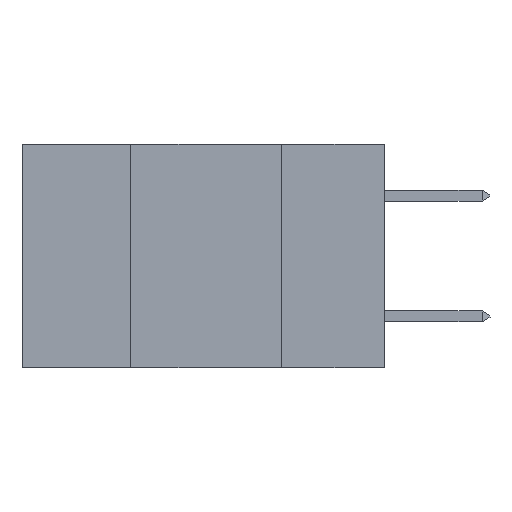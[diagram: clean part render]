
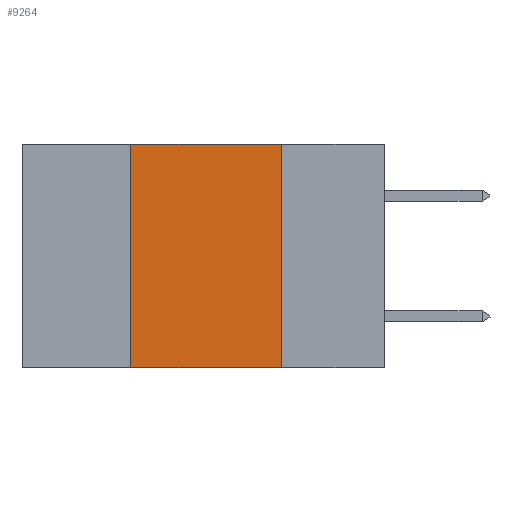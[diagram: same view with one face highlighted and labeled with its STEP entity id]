
A CAD part, left-side view. The second image highlights one B-rep face of the part: STEP entity #9264.
In plain terms, the highlighted planar face has unit normal (-1, 0, 0).
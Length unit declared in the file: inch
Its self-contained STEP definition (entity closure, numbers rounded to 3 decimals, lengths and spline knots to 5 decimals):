
#199 = ORIENTED_EDGE ( 'NONE', *, *, #4624, .F. ) ;
#1843 = CARTESIAN_POINT ( 'NONE',  ( 0., 0.6, 0. ) ) ;
#1872 = CARTESIAN_POINT ( 'NONE',  ( 0., 0.6, 0. ) ) ;
#2450 = VERTEX_POINT ( 'NONE', #16809 ) ;
#3179 = VECTOR ( 'NONE', #14970, 39.37008 ) ;
#3286 = ORIENTED_EDGE ( 'NONE', *, *, #17825, .F. ) ;
#4027 = LINE ( 'NONE', #6583, #3179 ) ;
#4624 = EDGE_CURVE ( 'NONE', #12736, #6586, #13359, .T. ) ;
#4851 = EDGE_CURVE ( 'NONE', #12736, #7540, #17727, .T. ) ;
#5351 = CARTESIAN_POINT ( 'NONE',  ( 0., 0.17, -0.37 ) ) ;
#5704 = LINE ( 'NONE', #1872, #9385 ) ;
#6222 = PLANE ( 'NONE',  #11294 ) ;
#6583 = CARTESIAN_POINT ( 'NONE',  ( 0., 0.17, 0. ) ) ;
#6586 = VERTEX_POINT ( 'NONE', #15947 ) ;
#6644 = CARTESIAN_POINT ( 'NONE',  ( 0., 0.6, -0.37 ) ) ;
#7540 = VERTEX_POINT ( 'NONE', #5351 ) ;
#7575 = DIRECTION ( 'NONE',  ( 0., 0., -1. ) ) ;
#7886 = DIRECTION ( 'NONE',  ( 0., 0., 1. ) ) ;
#8541 = CARTESIAN_POINT ( 'NONE',  ( 0., 0.42, 0. ) ) ;
#8892 = DIRECTION ( 'NONE',  ( 0., -1., 0. ) ) ;
#9264 = ADVANCED_FACE ( 'NONE', ( #11070 ), #6222, .F. ) ;
#9385 = VECTOR ( 'NONE', #8892, 39.37008 ) ;
#9632 = VECTOR ( 'NONE', #7886, 39.37008 ) ;
#9831 = VECTOR ( 'NONE', #15040, 39.37008 ) ;
#11070 = FACE_OUTER_BOUND ( 'NONE', #12857, .T. ) ;
#11294 = AXIS2_PLACEMENT_3D ( 'NONE', #1843, #15993, #7575 ) ;
#11961 = ORIENTED_EDGE ( 'NONE', *, *, #4851, .T. ) ;
#12736 = VERTEX_POINT ( 'NONE', #14483 ) ;
#12766 = EDGE_CURVE ( 'NONE', #6586, #2450, #5704, .T. ) ;
#12857 = EDGE_LOOP ( 'NONE', ( #3286, #18079, #199, #11961 ) ) ;
#13359 = LINE ( 'NONE', #8541, #9632 ) ;
#14483 = CARTESIAN_POINT ( 'NONE',  ( 0., 0.42, -0.37 ) ) ;
#14970 = DIRECTION ( 'NONE',  ( 0., 0., -1. ) ) ;
#15040 = DIRECTION ( 'NONE',  ( 0., -1., 0. ) ) ;
#15947 = CARTESIAN_POINT ( 'NONE',  ( 0., 0.42, 0. ) ) ;
#15993 = DIRECTION ( 'NONE',  ( 1., 0., 0. ) ) ;
#16809 = CARTESIAN_POINT ( 'NONE',  ( 0., 0.17, 0. ) ) ;
#17727 = LINE ( 'NONE', #6644, #9831 ) ;
#17825 = EDGE_CURVE ( 'NONE', #2450, #7540, #4027, .T. ) ;
#18079 = ORIENTED_EDGE ( 'NONE', *, *, #12766, .F. ) ;
